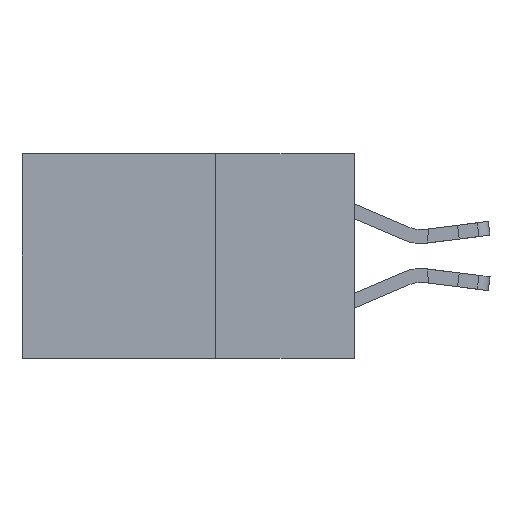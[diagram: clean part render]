
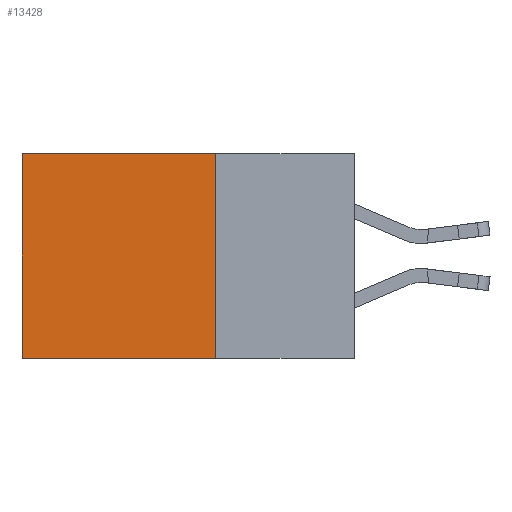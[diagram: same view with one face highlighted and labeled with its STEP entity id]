
A CAD part, left-side view. The second image highlights one B-rep face of the part: STEP entity #13428.
In plain terms, the highlighted planar face has unit normal (-1, 0, 0).
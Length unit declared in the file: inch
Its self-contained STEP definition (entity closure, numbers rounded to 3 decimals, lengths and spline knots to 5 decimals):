
#1024 = CARTESIAN_POINT ( 'NONE',  ( 0.298, 0.25, 0. ) ) ;
#1061 = LINE ( 'NONE', #1831, #12473 ) ;
#1437 = VERTEX_POINT ( 'NONE', #12783 ) ;
#1797 = CARTESIAN_POINT ( 'NONE',  ( 0.298, 0.6, -0.37 ) ) ;
#1831 = CARTESIAN_POINT ( 'NONE',  ( 0.298, 0.6, 0. ) ) ;
#1872 = EDGE_CURVE ( 'NONE', #1437, #2873, #1061, .T. ) ;
#2326 = EDGE_CURVE ( 'NONE', #6572, #2873, #11430, .T. ) ;
#2873 = VERTEX_POINT ( 'NONE', #1797 ) ;
#3258 = AXIS2_PLACEMENT_3D ( 'NONE', #5755, #3769, #11382 ) ;
#3426 = DIRECTION ( 'NONE',  ( 0., 0., -1. ) ) ;
#3769 = DIRECTION ( 'NONE',  ( 1., 0., 0. ) ) ;
#4748 = DIRECTION ( 'NONE',  ( 0., 1., 0. ) ) ;
#5184 = ORIENTED_EDGE ( 'NONE', *, *, #9630, .F. ) ;
#5190 = DIRECTION ( 'NONE',  ( 0., 0., -1. ) ) ;
#5388 = CARTESIAN_POINT ( 'NONE',  ( 0.298, 0.25, -0.37 ) ) ;
#5514 = CARTESIAN_POINT ( 'NONE',  ( 0.298, 0.25, 0. ) ) ;
#5755 = CARTESIAN_POINT ( 'NONE',  ( 0.298, 0.25, 0. ) ) ;
#6141 = FACE_OUTER_BOUND ( 'NONE', #13705, .T. ) ;
#6377 = DIRECTION ( 'NONE',  ( 0., 1., 0. ) ) ;
#6572 = VERTEX_POINT ( 'NONE', #5388 ) ;
#7155 = VECTOR ( 'NONE', #6377, 39.37008 ) ;
#7249 = EDGE_CURVE ( 'NONE', #8403, #1437, #12137, .T. ) ;
#7370 = ORIENTED_EDGE ( 'NONE', *, *, #7249, .T. ) ;
#8403 = VERTEX_POINT ( 'NONE', #1024 ) ;
#8432 = CARTESIAN_POINT ( 'NONE',  ( 0.298, 0.25, -0.37 ) ) ;
#8855 = LINE ( 'NONE', #5514, #13626 ) ;
#9515 = VECTOR ( 'NONE', #4748, 39.37008 ) ;
#9630 = EDGE_CURVE ( 'NONE', #8403, #6572, #8855, .T. ) ;
#10277 = PLANE ( 'NONE',  #3258 ) ;
#11382 = DIRECTION ( 'NONE',  ( 0., 0., -1. ) ) ;
#11430 = LINE ( 'NONE', #8432, #7155 ) ;
#11460 = ORIENTED_EDGE ( 'NONE', *, *, #2326, .F. ) ;
#12137 = LINE ( 'NONE', #13356, #9515 ) ;
#12473 = VECTOR ( 'NONE', #5190, 39.37008 ) ;
#12783 = CARTESIAN_POINT ( 'NONE',  ( 0.298, 0.6, 0. ) ) ;
#13356 = CARTESIAN_POINT ( 'NONE',  ( 0.298, 0.25, 0. ) ) ;
#13428 = ADVANCED_FACE ( 'NONE', ( #6141 ), #10277, .F. ) ;
#13544 = ORIENTED_EDGE ( 'NONE', *, *, #1872, .T. ) ;
#13626 = VECTOR ( 'NONE', #3426, 39.37008 ) ;
#13705 = EDGE_LOOP ( 'NONE', ( #13544, #11460, #5184, #7370 ) ) ;
